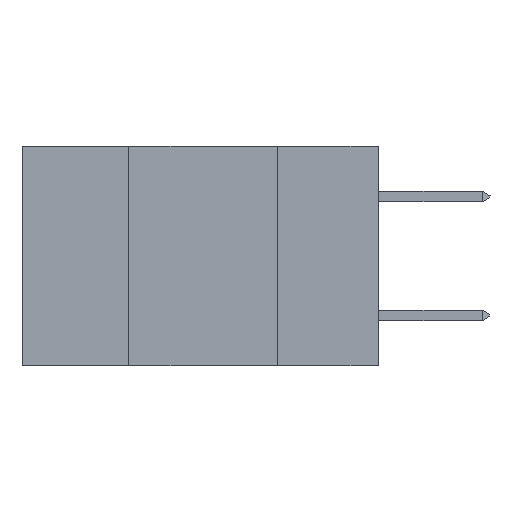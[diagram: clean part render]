
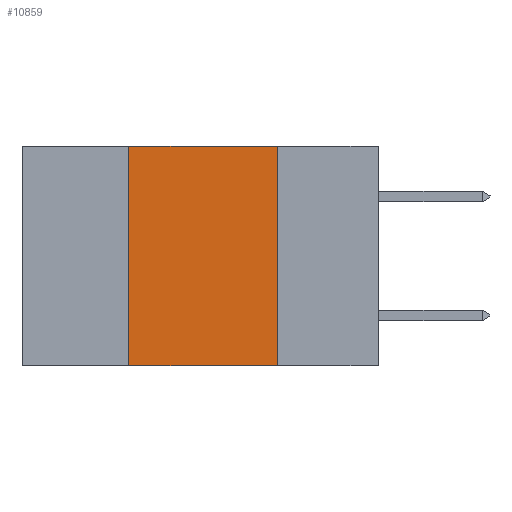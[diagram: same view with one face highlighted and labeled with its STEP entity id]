
A CAD part, left-side view. The second image highlights one B-rep face of the part: STEP entity #10859.
In plain terms, the highlighted planar face has unit normal (-1, 0, 0).
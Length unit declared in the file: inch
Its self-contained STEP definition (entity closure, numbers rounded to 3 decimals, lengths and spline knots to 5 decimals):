
#22 = DIRECTION ( 'NONE',  ( 0., 0., -1. ) ) ;
#53 = LINE ( 'NONE', #17399, #3623 ) ;
#1429 = LINE ( 'NONE', #13000, #16758 ) ;
#1759 = LINE ( 'NONE', #7560, #16976 ) ;
#2716 = DIRECTION ( 'NONE',  ( 1., 0., 0. ) ) ;
#2861 = ORIENTED_EDGE ( 'NONE', *, *, #14127, .F. ) ;
#3266 = DIRECTION ( 'NONE',  ( 0., 0., 1. ) ) ;
#3623 = VECTOR ( 'NONE', #3266, 39.37008 ) ;
#4539 = CARTESIAN_POINT ( 'NONE',  ( 0., 0.42, 0. ) ) ;
#4657 = CARTESIAN_POINT ( 'NONE',  ( 0., 0.42, -0.37 ) ) ;
#4921 = LINE ( 'NONE', #12225, #14941 ) ;
#5663 = CARTESIAN_POINT ( 'NONE',  ( 0., 0.6, 0. ) ) ;
#6977 = VERTEX_POINT ( 'NONE', #4657 ) ;
#7560 = CARTESIAN_POINT ( 'NONE',  ( 0., 0.6, -0.37 ) ) ;
#7848 = DIRECTION ( 'NONE',  ( 0., -1., 0. ) ) ;
#9556 = DIRECTION ( 'NONE',  ( 0., -1., 0. ) ) ;
#9850 = DIRECTION ( 'NONE',  ( 0., 0., -1. ) ) ;
#10089 = CARTESIAN_POINT ( 'NONE',  ( 0., 0.17, 0. ) ) ;
#10314 = VERTEX_POINT ( 'NONE', #15913 ) ;
#10360 = AXIS2_PLACEMENT_3D ( 'NONE', #5663, #2716, #9850 ) ;
#10585 = EDGE_CURVE ( 'NONE', #18404, #18027, #4921, .T. ) ;
#10859 = ADVANCED_FACE ( 'NONE', ( #18648 ), #14574, .F. ) ;
#12225 = CARTESIAN_POINT ( 'NONE',  ( 0., 0.6, 0. ) ) ;
#13000 = CARTESIAN_POINT ( 'NONE',  ( 0., 0.17, -0.37 ) ) ;
#14127 = EDGE_CURVE ( 'NONE', #6977, #18404, #53, .T. ) ;
#14530 = EDGE_LOOP ( 'NONE', ( #16351, #14902, #2861, #16461 ) ) ;
#14574 = PLANE ( 'NONE',  #10360 ) ;
#14902 = ORIENTED_EDGE ( 'NONE', *, *, #10585, .F. ) ;
#14941 = VECTOR ( 'NONE', #7848, 39.37008 ) ;
#15199 = EDGE_CURVE ( 'NONE', #6977, #10314, #1759, .T. ) ;
#15913 = CARTESIAN_POINT ( 'NONE',  ( 0., 0.17, -0.37 ) ) ;
#16351 = ORIENTED_EDGE ( 'NONE', *, *, #18035, .F. ) ;
#16461 = ORIENTED_EDGE ( 'NONE', *, *, #15199, .T. ) ;
#16758 = VECTOR ( 'NONE', #22, 39.37008 ) ;
#16976 = VECTOR ( 'NONE', #9556, 39.37008 ) ;
#17399 = CARTESIAN_POINT ( 'NONE',  ( 0., 0.42, -0.37 ) ) ;
#18027 = VERTEX_POINT ( 'NONE', #10089 ) ;
#18035 = EDGE_CURVE ( 'NONE', #18027, #10314, #1429, .T. ) ;
#18404 = VERTEX_POINT ( 'NONE', #4539 ) ;
#18648 = FACE_OUTER_BOUND ( 'NONE', #14530, .T. ) ;
